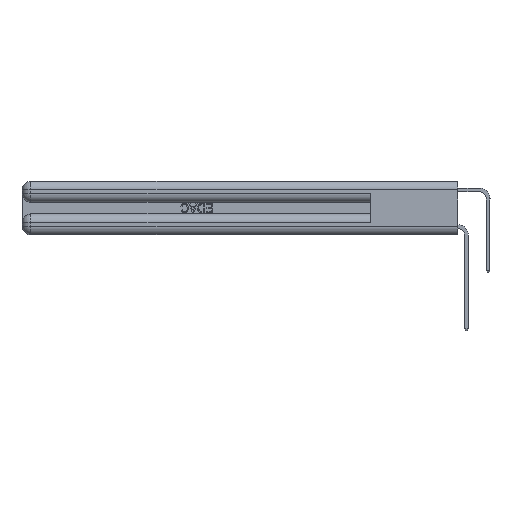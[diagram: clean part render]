
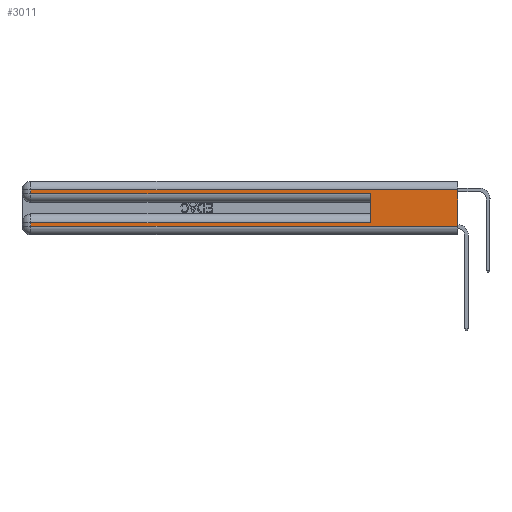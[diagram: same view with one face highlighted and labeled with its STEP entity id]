
A CAD part, left-side view. The second image highlights one B-rep face of the part: STEP entity #3011.
In plain terms, the highlighted planar face has unit normal (-1, 0, 0).
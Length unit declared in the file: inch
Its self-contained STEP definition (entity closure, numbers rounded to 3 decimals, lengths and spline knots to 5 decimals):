
#282 = VERTEX_POINT ( 'NONE', #818 ) ;
#818 = CARTESIAN_POINT ( 'NONE',  ( 0., 0., 0.31 ) ) ;
#850 = VECTOR ( 'NONE', #21870, 39.37008 ) ;
#1862 = CARTESIAN_POINT ( 'NONE',  ( 0., 2.94, 0.31 ) ) ;
#2156 = LINE ( 'NONE', #18959, #12574 ) ;
#2178 = CARTESIAN_POINT ( 'NONE',  ( 0., 2.94, 0.085 ) ) ;
#2701 = CARTESIAN_POINT ( 'NONE',  ( 0., 0., 0.085 ) ) ;
#2731 = CARTESIAN_POINT ( 'NONE',  ( 0., 0., 0.31 ) ) ;
#3011 = ADVANCED_FACE ( 'NONE', ( #13608 ), #19705, .F. ) ;
#3491 = EDGE_CURVE ( 'NONE', #26494, #15701, #27358, .T. ) ;
#4050 = CARTESIAN_POINT ( 'NONE',  ( 0., 0., 0.37 ) ) ;
#4755 = DIRECTION ( 'NONE',  ( 0., 0., 1. ) ) ;
#4783 = ORIENTED_EDGE ( 'NONE', *, *, #14080, .F. ) ;
#5264 = CARTESIAN_POINT ( 'NONE',  ( 0., 0., 0.06 ) ) ;
#5461 = DIRECTION ( 'NONE',  ( 1., 0., 0. ) ) ;
#5967 = VERTEX_POINT ( 'NONE', #18477 ) ;
#6608 = VECTOR ( 'NONE', #16997, 39.37008 ) ;
#7871 = DIRECTION ( 'NONE',  ( 0., 0., -1. ) ) ;
#8360 = VECTOR ( 'NONE', #16740, 39.37008 ) ;
#8611 = VECTOR ( 'NONE', #20694, 39.37008 ) ;
#8760 = VECTOR ( 'NONE', #18456, 39.37008 ) ;
#9822 = EDGE_CURVE ( 'NONE', #15191, #13807, #13317, .T. ) ;
#12324 = CARTESIAN_POINT ( 'NONE',  ( 0., 2.94, 0.06 ) ) ;
#12574 = VECTOR ( 'NONE', #4755, 39.37008 ) ;
#13070 = AXIS2_PLACEMENT_3D ( 'NONE', #15025, #5461, #7871 ) ;
#13317 = LINE ( 'NONE', #5264, #6608 ) ;
#13458 = LINE ( 'NONE', #2731, #19365 ) ;
#13608 = FACE_OUTER_BOUND ( 'NONE', #24078, .T. ) ;
#13807 = VERTEX_POINT ( 'NONE', #16502 ) ;
#14080 = EDGE_CURVE ( 'NONE', #282, #13807, #17482, .T. ) ;
#14332 = LINE ( 'NONE', #25588, #8760 ) ;
#15025 = CARTESIAN_POINT ( 'NONE',  ( 0., 0., 0.37 ) ) ;
#15191 = VERTEX_POINT ( 'NONE', #12324 ) ;
#15701 = VERTEX_POINT ( 'NONE', #17547 ) ;
#16093 = LINE ( 'NONE', #2701, #850 ) ;
#16502 = CARTESIAN_POINT ( 'NONE',  ( 0., 0., 0.06 ) ) ;
#16740 = DIRECTION ( 'NONE',  ( 0., 0., -1. ) ) ;
#16875 = VECTOR ( 'NONE', #21070, 39.37008 ) ;
#16997 = DIRECTION ( 'NONE',  ( 0., -1., 0. ) ) ;
#17482 = LINE ( 'NONE', #4050, #8611 ) ;
#17547 = CARTESIAN_POINT ( 'NONE',  ( 0., 2.94, 0.285 ) ) ;
#17621 = VERTEX_POINT ( 'NONE', #30034 ) ;
#17625 = LINE ( 'NONE', #27835, #16875 ) ;
#17959 = ORIENTED_EDGE ( 'NONE', *, *, #29014, .F. ) ;
#18456 = DIRECTION ( 'NONE',  ( 0., -1., 0. ) ) ;
#18477 = CARTESIAN_POINT ( 'NONE',  ( 0., 0.6, 0.285 ) ) ;
#18886 = VERTEX_POINT ( 'NONE', #2178 ) ;
#18959 = CARTESIAN_POINT ( 'NONE',  ( 0., 0.6, 0.145 ) ) ;
#19365 = VECTOR ( 'NONE', #21566, 39.37008 ) ;
#19705 = PLANE ( 'NONE',  #13070 ) ;
#19950 = ORIENTED_EDGE ( 'NONE', *, *, #3491, .T. ) ;
#20694 = DIRECTION ( 'NONE',  ( 0., 0., -1. ) ) ;
#21070 = DIRECTION ( 'NONE',  ( 0., 0., -1. ) ) ;
#21566 = DIRECTION ( 'NONE',  ( 0., 1., 0. ) ) ;
#21870 = DIRECTION ( 'NONE',  ( 0., 1., 0. ) ) ;
#22042 = ORIENTED_EDGE ( 'NONE', *, *, #30384, .T. ) ;
#23647 = EDGE_CURVE ( 'NONE', #18886, #15191, #17625, .T. ) ;
#24078 = EDGE_LOOP ( 'NONE', ( #4783, #28892, #19950, #22042, #17959, #26625, #24757, #26833 ) ) ;
#24306 = CARTESIAN_POINT ( 'NONE',  ( 0., 2.94, 0.37 ) ) ;
#24757 = ORIENTED_EDGE ( 'NONE', *, *, #23647, .T. ) ;
#25080 = EDGE_CURVE ( 'NONE', #17621, #18886, #16093, .T. ) ;
#25588 = CARTESIAN_POINT ( 'NONE',  ( 0., 0., 0.285 ) ) ;
#26103 = EDGE_CURVE ( 'NONE', #282, #26494, #13458, .T. ) ;
#26494 = VERTEX_POINT ( 'NONE', #1862 ) ;
#26625 = ORIENTED_EDGE ( 'NONE', *, *, #25080, .T. ) ;
#26833 = ORIENTED_EDGE ( 'NONE', *, *, #9822, .T. ) ;
#27358 = LINE ( 'NONE', #24306, #8360 ) ;
#27835 = CARTESIAN_POINT ( 'NONE',  ( 0., 2.94, 0.37 ) ) ;
#28892 = ORIENTED_EDGE ( 'NONE', *, *, #26103, .T. ) ;
#29014 = EDGE_CURVE ( 'NONE', #17621, #5967, #2156, .T. ) ;
#30034 = CARTESIAN_POINT ( 'NONE',  ( 0., 0.6, 0.085 ) ) ;
#30384 = EDGE_CURVE ( 'NONE', #15701, #5967, #14332, .T. ) ;
